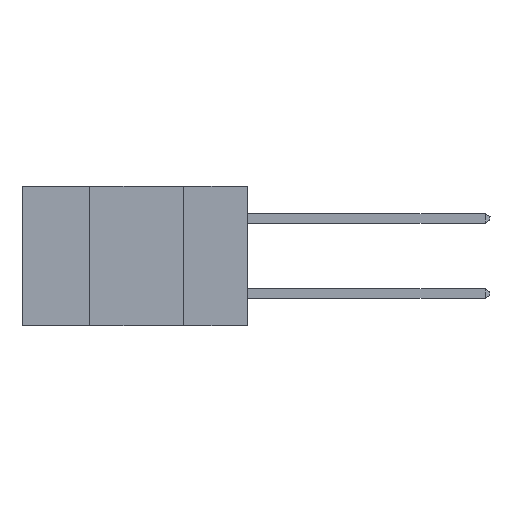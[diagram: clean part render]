
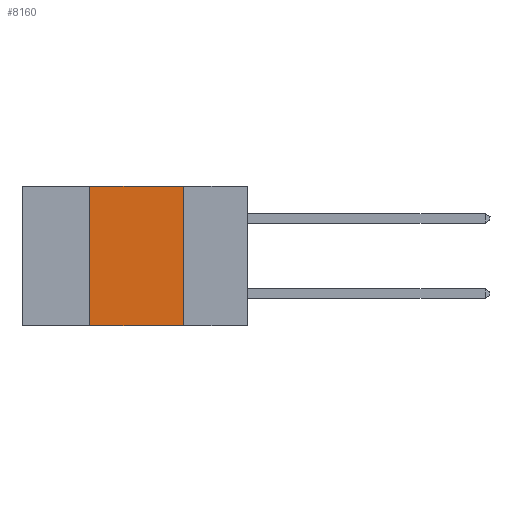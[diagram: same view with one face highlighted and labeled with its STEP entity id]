
A CAD part, left-side view. The second image highlights one B-rep face of the part: STEP entity #8160.
In plain terms, the highlighted planar face has unit normal (-1, 0, 0).
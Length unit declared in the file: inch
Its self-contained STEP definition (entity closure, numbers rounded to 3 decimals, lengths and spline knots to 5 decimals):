
#92 = DIRECTION ( 'NONE',  ( 0., 0., -1. ) ) ;
#339 = LINE ( 'NONE', #2454, #9176 ) ;
#833 = EDGE_CURVE ( 'NONE', #6585, #10647, #9234, .T. ) ;
#1206 = EDGE_CURVE ( 'NONE', #4535, #10647, #7000, .T. ) ;
#2364 = CARTESIAN_POINT ( 'NONE',  ( 0., 0.42, -0.37 ) ) ;
#2454 = CARTESIAN_POINT ( 'NONE',  ( 0., 0.6, 0. ) ) ;
#2901 = ORIENTED_EDGE ( 'NONE', *, *, #8264, .F. ) ;
#4031 = DIRECTION ( 'NONE',  ( 1., 0., 0. ) ) ;
#4079 = VERTEX_POINT ( 'NONE', #5146 ) ;
#4535 = VERTEX_POINT ( 'NONE', #12866 ) ;
#5030 = CARTESIAN_POINT ( 'NONE',  ( 0., 0.6, -0.37 ) ) ;
#5146 = CARTESIAN_POINT ( 'NONE',  ( 0., 0.42, 0. ) ) ;
#5802 = VECTOR ( 'NONE', #6404, 39.37008 ) ;
#5961 = ORIENTED_EDGE ( 'NONE', *, *, #9201, .F. ) ;
#6058 = PLANE ( 'NONE',  #6462 ) ;
#6296 = VECTOR ( 'NONE', #11321, 39.37008 ) ;
#6404 = DIRECTION ( 'NONE',  ( 0., 0., 1. ) ) ;
#6438 = DIRECTION ( 'NONE',  ( 0., -1., 0. ) ) ;
#6462 = AXIS2_PLACEMENT_3D ( 'NONE', #10956, #4031, #92 ) ;
#6585 = VERTEX_POINT ( 'NONE', #11427 ) ;
#6938 = DIRECTION ( 'NONE',  ( 0., -1., 0. ) ) ;
#7000 = LINE ( 'NONE', #5030, #10890 ) ;
#7045 = CARTESIAN_POINT ( 'NONE',  ( 0., 0.17, -0.37 ) ) ;
#7338 = CARTESIAN_POINT ( 'NONE',  ( 0., 0.17, -0.37 ) ) ;
#7605 = ORIENTED_EDGE ( 'NONE', *, *, #833, .F. ) ;
#8160 = ADVANCED_FACE ( 'NONE', ( #12874 ), #6058, .F. ) ;
#8264 = EDGE_CURVE ( 'NONE', #4079, #6585, #339, .T. ) ;
#8383 = LINE ( 'NONE', #2364, #5802 ) ;
#9176 = VECTOR ( 'NONE', #6438, 39.37008 ) ;
#9201 = EDGE_CURVE ( 'NONE', #4535, #4079, #8383, .T. ) ;
#9234 = LINE ( 'NONE', #7338, #6296 ) ;
#10137 = EDGE_LOOP ( 'NONE', ( #7605, #2901, #5961, #10514 ) ) ;
#10514 = ORIENTED_EDGE ( 'NONE', *, *, #1206, .T. ) ;
#10647 = VERTEX_POINT ( 'NONE', #7045 ) ;
#10890 = VECTOR ( 'NONE', #6938, 39.37008 ) ;
#10956 = CARTESIAN_POINT ( 'NONE',  ( 0., 0.6, 0. ) ) ;
#11321 = DIRECTION ( 'NONE',  ( 0., 0., -1. ) ) ;
#11427 = CARTESIAN_POINT ( 'NONE',  ( 0., 0.17, 0. ) ) ;
#12866 = CARTESIAN_POINT ( 'NONE',  ( 0., 0.42, -0.37 ) ) ;
#12874 = FACE_OUTER_BOUND ( 'NONE', #10137, .T. ) ;
